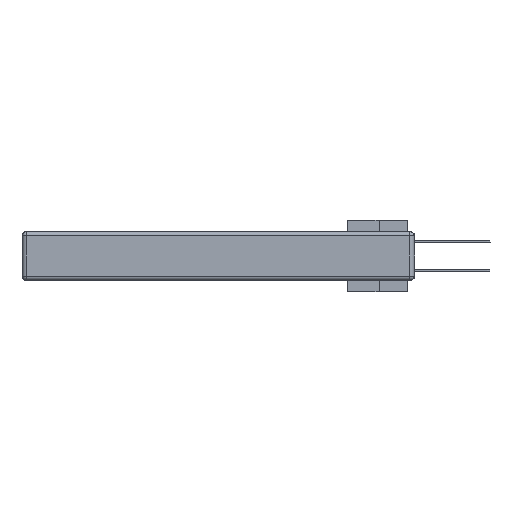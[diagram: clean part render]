
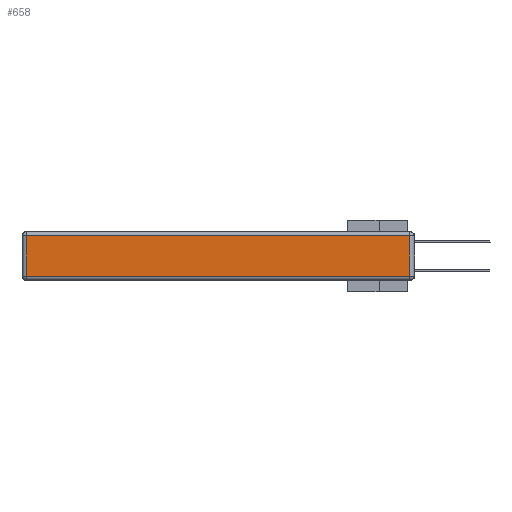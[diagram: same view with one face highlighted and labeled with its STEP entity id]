
A CAD part, left-side view. The second image highlights one B-rep face of the part: STEP entity #658.
In plain terms, the highlighted planar face has unit normal (-1, 0, 0).
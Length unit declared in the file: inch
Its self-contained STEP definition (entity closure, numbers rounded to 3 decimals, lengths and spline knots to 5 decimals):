
#353 = LINE ( 'NONE', #35109, #39186 ) ;
#658 = ADVANCED_FACE ( 'NONE', ( #20652 ), #17354, .T. ) ;
#1804 = DIRECTION ( 'NONE',  ( 0., 1., 0. ) ) ;
#1815 = DIRECTION ( 'NONE',  ( -1., 0., 0. ) ) ;
#2334 = ORIENTED_EDGE ( 'NONE', *, *, #33595, .T. ) ;
#3343 = VERTEX_POINT ( 'NONE', #37914 ) ;
#3931 = VECTOR ( 'NONE', #13979, 39.37008 ) ;
#4033 = CARTESIAN_POINT ( 'NONE',  ( 0., 0., -0.313 ) ) ;
#4297 = LINE ( 'NONE', #19833, #23160 ) ;
#9158 = ORIENTED_EDGE ( 'NONE', *, *, #13265, .T. ) ;
#10933 = DIRECTION ( 'NONE',  ( 0., 0., 1. ) ) ;
#12231 = CARTESIAN_POINT ( 'NONE',  ( 0., 0.03, -0.03 ) ) ;
#12697 = CARTESIAN_POINT ( 'NONE',  ( 0., 2.72, -0.343 ) ) ;
#13265 = EDGE_CURVE ( 'NONE', #19139, #3343, #4297, .T. ) ;
#13979 = DIRECTION ( 'NONE',  ( 0., -1., 0. ) ) ;
#14045 = CARTESIAN_POINT ( 'NONE',  ( 0., 0., -0.343 ) ) ;
#16848 = AXIS2_PLACEMENT_3D ( 'NONE', #14045, #1815, #10933 ) ;
#17354 = PLANE ( 'NONE',  #16848 ) ;
#17985 = EDGE_LOOP ( 'NONE', ( #2334, #29726, #9158, #38771 ) ) ;
#19139 = VERTEX_POINT ( 'NONE', #12231 ) ;
#19372 = DIRECTION ( 'NONE',  ( 0., 0., 1. ) ) ;
#19833 = CARTESIAN_POINT ( 'NONE',  ( 0., 2.75, -0.03 ) ) ;
#20652 = FACE_OUTER_BOUND ( 'NONE', #17985, .T. ) ;
#23160 = VECTOR ( 'NONE', #1804, 39.37008 ) ;
#25264 = CARTESIAN_POINT ( 'NONE',  ( 0., 0.03, -0.313 ) ) ;
#25298 = DIRECTION ( 'NONE',  ( 0., 0., -1. ) ) ;
#25439 = VERTEX_POINT ( 'NONE', #38742 ) ;
#25553 = EDGE_CURVE ( 'NONE', #3343, #25439, #37925, .T. ) ;
#28410 = VERTEX_POINT ( 'NONE', #25264 ) ;
#29726 = ORIENTED_EDGE ( 'NONE', *, *, #36816, .T. ) ;
#33595 = EDGE_CURVE ( 'NONE', #25439, #28410, #38398, .T. ) ;
#35109 = CARTESIAN_POINT ( 'NONE',  ( 0., 0.03, -0.343 ) ) ;
#36816 = EDGE_CURVE ( 'NONE', #28410, #19139, #353, .T. ) ;
#37914 = CARTESIAN_POINT ( 'NONE',  ( 0., 2.72, -0.03 ) ) ;
#37925 = LINE ( 'NONE', #12697, #38006 ) ;
#38006 = VECTOR ( 'NONE', #25298, 39.37008 ) ;
#38398 = LINE ( 'NONE', #4033, #3931 ) ;
#38742 = CARTESIAN_POINT ( 'NONE',  ( 0., 2.72, -0.313 ) ) ;
#38771 = ORIENTED_EDGE ( 'NONE', *, *, #25553, .T. ) ;
#39186 = VECTOR ( 'NONE', #19372, 39.37008 ) ;
